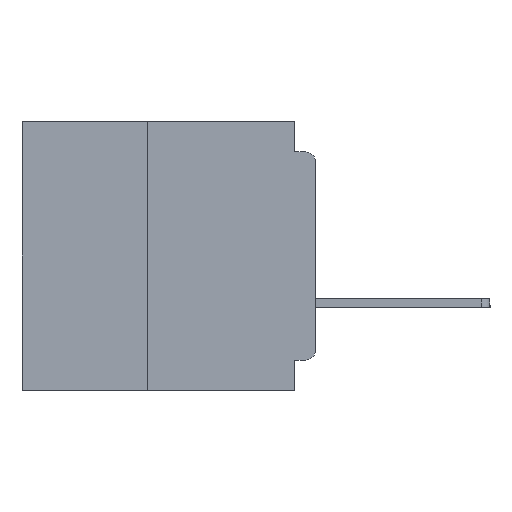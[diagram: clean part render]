
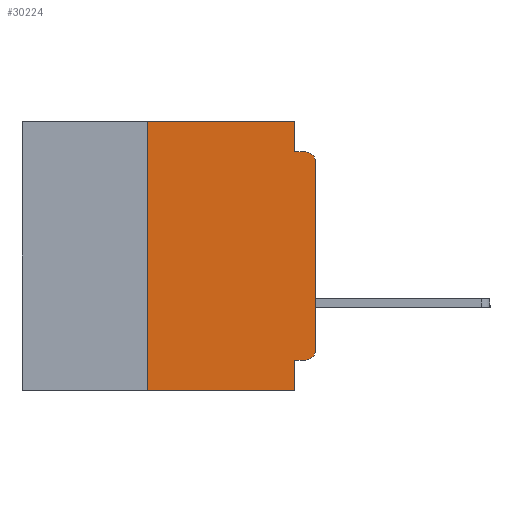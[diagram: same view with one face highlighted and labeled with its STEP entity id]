
A CAD part, left-side view. The second image highlights one B-rep face of the part: STEP entity #30224.
In plain terms, the highlighted planar face has unit normal (-1, 0, 0).
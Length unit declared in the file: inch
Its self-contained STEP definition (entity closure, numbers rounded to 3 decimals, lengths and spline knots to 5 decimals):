
#285 = DIRECTION ( 'NONE',  ( 0., 0., -1. ) ) ;
#1350 = CARTESIAN_POINT ( 'NONE',  ( 0., 0.25, 0. ) ) ;
#1548 = DIRECTION ( 'NONE',  ( 0., 0., 1. ) ) ;
#1793 = DIRECTION ( 'NONE',  ( 0., 0., -1. ) ) ;
#2639 = ORIENTED_EDGE ( 'NONE', *, *, #41174, .T. ) ;
#3222 = VECTOR ( 'NONE', #21693, 39.37008 ) ;
#3242 = DIRECTION ( 'NONE',  ( -1., 0., 0. ) ) ;
#3776 = VERTEX_POINT ( 'NONE', #52621 ) ;
#4441 = VECTOR ( 'NONE', #9950, 39.37008 ) ;
#4566 = LINE ( 'NONE', #49780, #51615 ) ;
#6513 = CIRCLE ( 'NONE', #46246, 0.015 ) ;
#7280 = DIRECTION ( 'NONE',  ( 0., 0., -1. ) ) ;
#7740 = EDGE_CURVE ( 'NONE', #37132, #14969, #16760, .T. ) ;
#8295 = VECTOR ( 'NONE', #1548, 39.37008 ) ;
#9418 = LINE ( 'NONE', #32604, #32527 ) ;
#9950 = DIRECTION ( 'NONE',  ( 0., -1., 0. ) ) ;
#10649 = ORIENTED_EDGE ( 'NONE', *, *, #51423, .F. ) ;
#12027 = ORIENTED_EDGE ( 'NONE', *, *, #16118, .T. ) ;
#12841 = ORIENTED_EDGE ( 'NONE', *, *, #31357, .F. ) ;
#13277 = VERTEX_POINT ( 'NONE', #57748 ) ;
#14419 = CARTESIAN_POINT ( 'NONE',  ( 0., 0.031, -0.045 ) ) ;
#14969 = VERTEX_POINT ( 'NONE', #20096 ) ;
#16118 = EDGE_CURVE ( 'NONE', #37613, #28572, #20612, .T. ) ;
#16273 = AXIS2_PLACEMENT_3D ( 'NONE', #56332, #29519, #1793 ) ;
#16461 = ORIENTED_EDGE ( 'NONE', *, *, #52891, .F. ) ;
#16760 = LINE ( 'NONE', #28354, #4441 ) ;
#16876 = ORIENTED_EDGE ( 'NONE', *, *, #7740, .F. ) ;
#17472 = EDGE_CURVE ( 'NONE', #53372, #42180, #56452, .T. ) ;
#18622 = CIRCLE ( 'NONE', #16273, 0.015 ) ;
#20096 = CARTESIAN_POINT ( 'NONE',  ( 0., 0.015, -0.045 ) ) ;
#20612 = LINE ( 'NONE', #29267, #8295 ) ;
#21693 = DIRECTION ( 'NONE',  ( 0., -1., 0. ) ) ;
#21861 = ORIENTED_EDGE ( 'NONE', *, *, #54843, .T. ) ;
#22000 = EDGE_CURVE ( 'NONE', #13277, #41124, #34541, .T. ) ;
#22158 = ORIENTED_EDGE ( 'NONE', *, *, #47570, .F. ) ;
#22181 = PLANE ( 'NONE',  #31950 ) ;
#26355 = LINE ( 'NONE', #48792, #3222 ) ;
#26814 = CARTESIAN_POINT ( 'NONE',  ( 0., 0.437, 0. ) ) ;
#27326 = DIRECTION ( 'NONE',  ( 0., 0., 1. ) ) ;
#28132 = DIRECTION ( 'NONE',  ( 0., -1., 0. ) ) ;
#28354 = CARTESIAN_POINT ( 'NONE',  ( 0., 0., -0.045 ) ) ;
#28572 = VERTEX_POINT ( 'NONE', #56124 ) ;
#29267 = CARTESIAN_POINT ( 'NONE',  ( 0., 0., 0. ) ) ;
#29519 = DIRECTION ( 'NONE',  ( -1., 0., 0. ) ) ;
#30224 = ADVANCED_FACE ( 'NONE', ( #37490 ), #22181, .F. ) ;
#30905 = CARTESIAN_POINT ( 'NONE',  ( 0., 0.015, -0.34 ) ) ;
#31357 = EDGE_CURVE ( 'NONE', #3776, #37132, #32265, .T. ) ;
#31427 = DIRECTION ( 'NONE',  ( 0., 0., -1. ) ) ;
#31950 = AXIS2_PLACEMENT_3D ( 'NONE', #26814, #58213, #31427 ) ;
#32265 = LINE ( 'NONE', #52653, #42722 ) ;
#32398 = ORIENTED_EDGE ( 'NONE', *, *, #22000, .T. ) ;
#32527 = VECTOR ( 'NONE', #285, 39.37008 ) ;
#32604 = CARTESIAN_POINT ( 'NONE',  ( 0., 0.031, -0.4 ) ) ;
#34541 = LINE ( 'NONE', #54995, #56934 ) ;
#35402 = DIRECTION ( 'NONE',  ( 0., 0., -1. ) ) ;
#36224 = ORIENTED_EDGE ( 'NONE', *, *, #17472, .F. ) ;
#37132 = VERTEX_POINT ( 'NONE', #14419 ) ;
#37490 = FACE_OUTER_BOUND ( 'NONE', #37588, .T. ) ;
#37588 = EDGE_LOOP ( 'NONE', ( #12027, #21861, #16876, #12841, #10649, #16461, #32398, #22158, #36224, #2639 ) ) ;
#37613 = VERTEX_POINT ( 'NONE', #54383 ) ;
#38741 = DIRECTION ( 'NONE',  ( 0., 1., 0. ) ) ;
#41124 = VERTEX_POINT ( 'NONE', #57116 ) ;
#41174 = EDGE_CURVE ( 'NONE', #53372, #37613, #6513, .T. ) ;
#42180 = VERTEX_POINT ( 'NONE', #55804 ) ;
#42722 = VECTOR ( 'NONE', #7280, 39.37008 ) ;
#44031 = VERTEX_POINT ( 'NONE', #1350 ) ;
#44358 = CARTESIAN_POINT ( 'NONE',  ( 0., 0.015, -0.355 ) ) ;
#44533 = VECTOR ( 'NONE', #38741, 39.37008 ) ;
#46246 = AXIS2_PLACEMENT_3D ( 'NONE', #30905, #3242, #35402 ) ;
#47570 = EDGE_CURVE ( 'NONE', #42180, #41124, #9418, .T. ) ;
#48792 = CARTESIAN_POINT ( 'NONE',  ( 0., 0.437, 0. ) ) ;
#49780 = CARTESIAN_POINT ( 'NONE',  ( 0., 0.25, -0.4 ) ) ;
#51423 = EDGE_CURVE ( 'NONE', #44031, #3776, #26355, .T. ) ;
#51615 = VECTOR ( 'NONE', #27326, 39.37008 ) ;
#52084 = CARTESIAN_POINT ( 'NONE',  ( 0., 0., -0.355 ) ) ;
#52621 = CARTESIAN_POINT ( 'NONE',  ( 0., 0.031, 0. ) ) ;
#52653 = CARTESIAN_POINT ( 'NONE',  ( 0., 0.031, 0. ) ) ;
#52891 = EDGE_CURVE ( 'NONE', #13277, #44031, #4566, .T. ) ;
#53372 = VERTEX_POINT ( 'NONE', #44358 ) ;
#54383 = CARTESIAN_POINT ( 'NONE',  ( 0., 0., -0.34 ) ) ;
#54843 = EDGE_CURVE ( 'NONE', #28572, #14969, #18622, .T. ) ;
#54995 = CARTESIAN_POINT ( 'NONE',  ( 0., 0.437, -0.4 ) ) ;
#55804 = CARTESIAN_POINT ( 'NONE',  ( 0., 0.031, -0.355 ) ) ;
#56124 = CARTESIAN_POINT ( 'NONE',  ( 0., 0., -0.06 ) ) ;
#56332 = CARTESIAN_POINT ( 'NONE',  ( 0., 0.015, -0.06 ) ) ;
#56452 = LINE ( 'NONE', #52084, #44533 ) ;
#56934 = VECTOR ( 'NONE', #28132, 39.37008 ) ;
#57116 = CARTESIAN_POINT ( 'NONE',  ( 0., 0.031, -0.4 ) ) ;
#57748 = CARTESIAN_POINT ( 'NONE',  ( 0., 0.25, -0.4 ) ) ;
#58213 = DIRECTION ( 'NONE',  ( 1., 0., 0. ) ) ;
